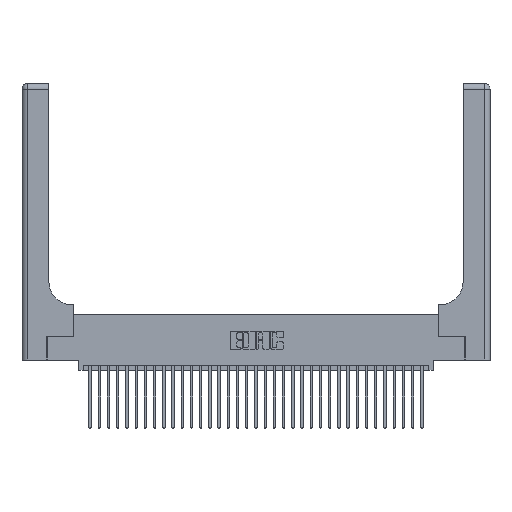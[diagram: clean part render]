
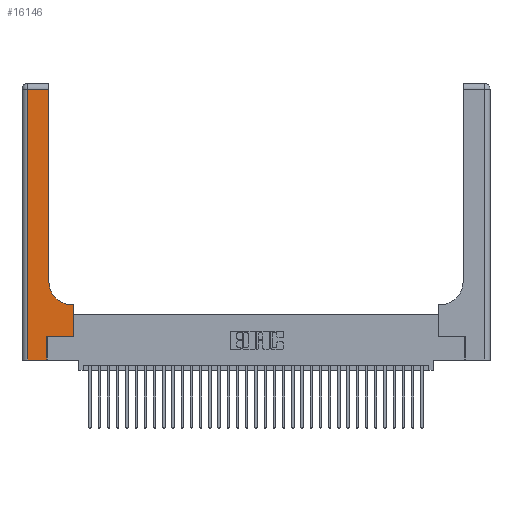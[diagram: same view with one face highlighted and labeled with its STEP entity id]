
A CAD part, top view. The second image highlights one B-rep face of the part: STEP entity #16146.
In plain terms, the highlighted planar face has unit normal (0, 0, 1).
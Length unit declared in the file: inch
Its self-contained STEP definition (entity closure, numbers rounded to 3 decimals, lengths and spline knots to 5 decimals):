
#1013 = CARTESIAN_POINT ( 'NONE',  ( 0.5415, 0.85, 0.37 ) ) ;
#1228 = DIRECTION ( 'NONE',  ( 0., 1., 0. ) ) ;
#2578 = DIRECTION ( 'NONE',  ( 1., 0., 0. ) ) ;
#2761 = CARTESIAN_POINT ( 'NONE',  ( 0.5585, 0.25, 0.37 ) ) ;
#2931 = DIRECTION ( 'NONE',  ( -1., 0., 0. ) ) ;
#3409 = CARTESIAN_POINT ( 'NONE',  ( 0., 3., 0.37 ) ) ;
#3566 = VERTEX_POINT ( 'NONE', #21548 ) ;
#3605 = DIRECTION ( 'NONE',  ( 0., -1., 0. ) ) ;
#3878 = DIRECTION ( 'NONE',  ( 1., 0., 0. ) ) ;
#4423 = VECTOR ( 'NONE', #1228, 39.37008 ) ;
#4929 = ORIENTED_EDGE ( 'NONE', *, *, #6268, .T. ) ;
#4935 = CARTESIAN_POINT ( 'NONE',  ( 0.2915, 2.94, 0.37 ) ) ;
#5381 = ORIENTED_EDGE ( 'NONE', *, *, #20437, .T. ) ;
#5589 = DIRECTION ( 'NONE',  ( 0., 1., 0. ) ) ;
#5803 = CARTESIAN_POINT ( 'NONE',  ( 0.06, 2.94, 0.37 ) ) ;
#6235 = DIRECTION ( 'NONE',  ( -1., 0., 0. ) ) ;
#6268 = EDGE_CURVE ( 'NONE', #32367, #11830, #20013, .T. ) ;
#6345 = VERTEX_POINT ( 'NONE', #32533 ) ;
#7009 = VECTOR ( 'NONE', #2578, 39.37008 ) ;
#7081 = LINE ( 'NONE', #19869, #26821 ) ;
#7357 = ORIENTED_EDGE ( 'NONE', *, *, #8559, .T. ) ;
#7847 = LINE ( 'NONE', #21915, #30093 ) ;
#8060 = VECTOR ( 'NONE', #33320, 39.37008 ) ;
#8559 = EDGE_CURVE ( 'NONE', #8898, #6345, #22345, .T. ) ;
#8898 = VERTEX_POINT ( 'NONE', #13297 ) ;
#9453 = VERTEX_POINT ( 'NONE', #5803 ) ;
#9658 = DIRECTION ( 'NONE',  ( 1., 0., 0. ) ) ;
#10124 = VECTOR ( 'NONE', #5589, 39.37008 ) ;
#10156 = VERTEX_POINT ( 'NONE', #32535 ) ;
#11161 = ORIENTED_EDGE ( 'NONE', *, *, #29199, .T. ) ;
#11191 = LINE ( 'NONE', #20361, #16612 ) ;
#11516 = AXIS2_PLACEMENT_3D ( 'NONE', #1013, #20108, #3878 ) ;
#11830 = VERTEX_POINT ( 'NONE', #33522 ) ;
#12209 = CARTESIAN_POINT ( 'NONE',  ( 0.2915, 3., 0.37 ) ) ;
#13297 = CARTESIAN_POINT ( 'NONE',  ( 0.269, 0., 0.37 ) ) ;
#13374 = LINE ( 'NONE', #12209, #4423 ) ;
#15336 = ORIENTED_EDGE ( 'NONE', *, *, #17954, .T. ) ;
#16146 = ADVANCED_FACE ( 'NONE', ( #34028 ), #32974, .F. ) ;
#16384 = DIRECTION ( 'NONE',  ( -1., 0., 0. ) ) ;
#16612 = VECTOR ( 'NONE', #9658, 39.37008 ) ;
#17954 = EDGE_CURVE ( 'NONE', #9453, #3566, #7081, .T. ) ;
#19104 = EDGE_CURVE ( 'NONE', #29471, #9453, #7847, .T. ) ;
#19156 = VECTOR ( 'NONE', #16384, 39.37008 ) ;
#19858 = EDGE_LOOP ( 'NONE', ( #11161, #19987, #15336, #20840, #7357, #23789, #27196, #4929, #5381 ) ) ;
#19869 = CARTESIAN_POINT ( 'NONE',  ( 0.06, 3., 0.37 ) ) ;
#19893 = EDGE_CURVE ( 'NONE', #3566, #8898, #11191, .T. ) ;
#19987 = ORIENTED_EDGE ( 'NONE', *, *, #19104, .T. ) ;
#20013 = LINE ( 'NONE', #24341, #19156 ) ;
#20108 = DIRECTION ( 'NONE',  ( 0., 0., -1. ) ) ;
#20361 = CARTESIAN_POINT ( 'NONE',  ( 0., 0., 0.37 ) ) ;
#20367 = CIRCLE ( 'NONE', #11516, 0.25 ) ;
#20437 = EDGE_CURVE ( 'NONE', #11830, #10156, #20367, .T. ) ;
#20840 = ORIENTED_EDGE ( 'NONE', *, *, #19893, .T. ) ;
#21548 = CARTESIAN_POINT ( 'NONE',  ( 0.06, 0., 0.37 ) ) ;
#21915 = CARTESIAN_POINT ( 'NONE',  ( 0., 2.94, 0.37 ) ) ;
#22345 = LINE ( 'NONE', #22578, #8060 ) ;
#22357 = DIRECTION ( 'NONE',  ( 0., 0., -1. ) ) ;
#22578 = CARTESIAN_POINT ( 'NONE',  ( 0.269, 0., 0.37 ) ) ;
#22770 = CARTESIAN_POINT ( 'NONE',  ( 0.5585, 0.6, 0.37 ) ) ;
#23271 = CARTESIAN_POINT ( 'NONE',  ( 0.5585, 0.25, 0.37 ) ) ;
#23789 = ORIENTED_EDGE ( 'NONE', *, *, #29558, .T. ) ;
#23820 = LINE ( 'NONE', #26815, #7009 ) ;
#24341 = CARTESIAN_POINT ( 'NONE',  ( 0.2915, 0.6, 0.37 ) ) ;
#25339 = EDGE_CURVE ( 'NONE', #28003, #32367, #31482, .T. ) ;
#26815 = CARTESIAN_POINT ( 'NONE',  ( 0.269, 0.25, 0.37 ) ) ;
#26821 = VECTOR ( 'NONE', #3605, 39.37008 ) ;
#27196 = ORIENTED_EDGE ( 'NONE', *, *, #25339, .T. ) ;
#28003 = VERTEX_POINT ( 'NONE', #23271 ) ;
#29199 = EDGE_CURVE ( 'NONE', #10156, #29471, #13374, .T. ) ;
#29471 = VERTEX_POINT ( 'NONE', #4935 ) ;
#29558 = EDGE_CURVE ( 'NONE', #6345, #28003, #23820, .T. ) ;
#30093 = VECTOR ( 'NONE', #2931, 39.37008 ) ;
#31482 = LINE ( 'NONE', #2761, #10124 ) ;
#32367 = VERTEX_POINT ( 'NONE', #22770 ) ;
#32533 = CARTESIAN_POINT ( 'NONE',  ( 0.269, 0.25, 0.37 ) ) ;
#32535 = CARTESIAN_POINT ( 'NONE',  ( 0.2915, 0.85, 0.37 ) ) ;
#32974 = PLANE ( 'NONE',  #33819 ) ;
#33320 = DIRECTION ( 'NONE',  ( 0., 1., 0. ) ) ;
#33522 = CARTESIAN_POINT ( 'NONE',  ( 0.5415, 0.6, 0.37 ) ) ;
#33819 = AXIS2_PLACEMENT_3D ( 'NONE', #3409, #22357, #6235 ) ;
#34028 = FACE_OUTER_BOUND ( 'NONE', #19858, .T. ) ;
